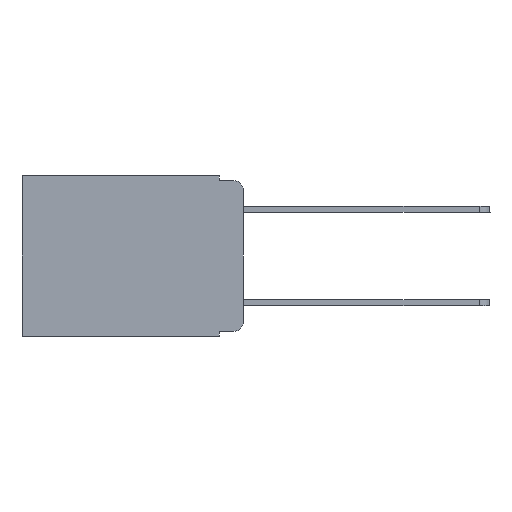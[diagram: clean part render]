
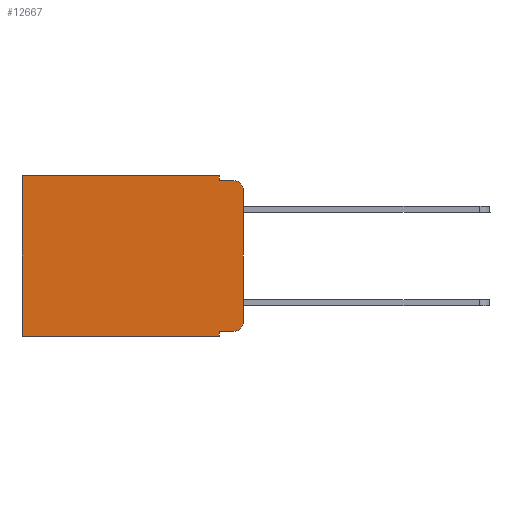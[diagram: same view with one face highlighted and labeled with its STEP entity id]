
A CAD part, left-side view. The second image highlights one B-rep face of the part: STEP entity #12667.
In plain terms, the highlighted planar face has unit normal (-1, 0, 0).
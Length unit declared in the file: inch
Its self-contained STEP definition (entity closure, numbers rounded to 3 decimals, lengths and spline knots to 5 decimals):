
#111 = CIRCLE ( 'NONE', #2934, 0.02 ) ;
#188 = ORIENTED_EDGE ( 'NONE', *, *, #13319, .T. ) ;
#190 = CIRCLE ( 'NONE', #20219, 0.02 ) ;
#275 = LINE ( 'NONE', #2709, #3419 ) ;
#318 = VERTEX_POINT ( 'NONE', #12634 ) ;
#684 = CARTESIAN_POINT ( 'NONE',  ( 0.298, 0.051, -0.333 ) ) ;
#744 = EDGE_CURVE ( 'NONE', #5972, #11045, #20165, .T. ) ;
#1204 = VECTOR ( 'NONE', #13060, 39.37008 ) ;
#1580 = CARTESIAN_POINT ( 'NONE',  ( 0.298, 0.051, 0. ) ) ;
#1635 = CARTESIAN_POINT ( 'NONE',  ( 0.298, 0., -0.343 ) ) ;
#1804 = DIRECTION ( 'NONE',  ( 0., 0., -1. ) ) ;
#1850 = LINE ( 'NONE', #1635, #4973 ) ;
#1986 = VERTEX_POINT ( 'NONE', #684 ) ;
#2709 = CARTESIAN_POINT ( 'NONE',  ( 0.298, 0.051, -0.333 ) ) ;
#2934 = AXIS2_PLACEMENT_3D ( 'NONE', #17163, #17082, #4686 ) ;
#3065 = CARTESIAN_POINT ( 'NONE',  ( 0.298, 0.02, -0.01 ) ) ;
#3326 = CARTESIAN_POINT ( 'NONE',  ( 0.298, 0., 0. ) ) ;
#3419 = VECTOR ( 'NONE', #6190, 39.37008 ) ;
#4187 = EDGE_CURVE ( 'NONE', #19024, #15727, #15552, .T. ) ;
#4202 = VECTOR ( 'NONE', #8834, 39.37008 ) ;
#4479 = FACE_OUTER_BOUND ( 'NONE', #5883, .T. ) ;
#4686 = DIRECTION ( 'NONE',  ( 0., 0., -1. ) ) ;
#4766 = AXIS2_PLACEMENT_3D ( 'NONE', #19698, #8995, #1804 ) ;
#4973 = VECTOR ( 'NONE', #15931, 39.37008 ) ;
#5771 = EDGE_CURVE ( 'NONE', #1986, #19850, #275, .T. ) ;
#5883 = EDGE_LOOP ( 'NONE', ( #16568, #188, #13346, #12240, #8488, #14328, #14435, #6673, #20327, #23247 ) ) ;
#5972 = VERTEX_POINT ( 'NONE', #1580 ) ;
#6190 = DIRECTION ( 'NONE',  ( 0., -1., 0. ) ) ;
#6331 = EDGE_CURVE ( 'NONE', #5972, #19024, #22505, .T. ) ;
#6673 = ORIENTED_EDGE ( 'NONE', *, *, #8323, .F. ) ;
#6708 = EDGE_CURVE ( 'NONE', #20943, #9662, #15771, .T. ) ;
#6944 = DIRECTION ( 'NONE',  ( 0., 0., -1. ) ) ;
#7244 = DIRECTION ( 'NONE',  ( 0., 0., -1. ) ) ;
#7416 = CARTESIAN_POINT ( 'NONE',  ( 0.298, 0., -0.313 ) ) ;
#7608 = CARTESIAN_POINT ( 'NONE',  ( 0.298, 0.473, 0. ) ) ;
#8323 = EDGE_CURVE ( 'NONE', #1986, #12819, #11779, .T. ) ;
#8488 = ORIENTED_EDGE ( 'NONE', *, *, #744, .T. ) ;
#8834 = DIRECTION ( 'NONE',  ( 0., 1., 0. ) ) ;
#8995 = DIRECTION ( 'NONE',  ( 1., 0., 0. ) ) ;
#9658 = CARTESIAN_POINT ( 'NONE',  ( 0.298, 0.051, -0.343 ) ) ;
#9662 = VERTEX_POINT ( 'NONE', #7416 ) ;
#10118 = DIRECTION ( 'NONE',  ( 0., 0., -1. ) ) ;
#10312 = EDGE_CURVE ( 'NONE', #12819, #318, #1850, .T. ) ;
#11045 = VERTEX_POINT ( 'NONE', #13282 ) ;
#11590 = VECTOR ( 'NONE', #7244, 39.37008 ) ;
#11779 = LINE ( 'NONE', #19026, #13176 ) ;
#12222 = CARTESIAN_POINT ( 'NONE',  ( 0.298, 0.051, -0.01 ) ) ;
#12240 = ORIENTED_EDGE ( 'NONE', *, *, #6331, .F. ) ;
#12578 = DIRECTION ( 'NONE',  ( -1., 0., 0. ) ) ;
#12582 = PLANE ( 'NONE',  #4766 ) ;
#12634 = CARTESIAN_POINT ( 'NONE',  ( 0.298, 0.473, -0.343 ) ) ;
#12667 = ADVANCED_FACE ( 'NONE', ( #4479 ), #12582, .F. ) ;
#12782 = DIRECTION ( 'NONE',  ( 0., 0., -1. ) ) ;
#12819 = VERTEX_POINT ( 'NONE', #9658 ) ;
#13060 = DIRECTION ( 'NONE',  ( 0., -1., 0. ) ) ;
#13176 = VECTOR ( 'NONE', #10118, 39.37008 ) ;
#13263 = VECTOR ( 'NONE', #15319, 39.37008 ) ;
#13282 = CARTESIAN_POINT ( 'NONE',  ( 0.298, 0.473, 0. ) ) ;
#13319 = EDGE_CURVE ( 'NONE', #20943, #15727, #190, .T. ) ;
#13346 = ORIENTED_EDGE ( 'NONE', *, *, #4187, .F. ) ;
#13872 = VECTOR ( 'NONE', #12782, 39.37008 ) ;
#14328 = ORIENTED_EDGE ( 'NONE', *, *, #16664, .T. ) ;
#14435 = ORIENTED_EDGE ( 'NONE', *, *, #10312, .F. ) ;
#15319 = DIRECTION ( 'NONE',  ( 0., 0., -1. ) ) ;
#15552 = LINE ( 'NONE', #18535, #1204 ) ;
#15727 = VERTEX_POINT ( 'NONE', #3065 ) ;
#15771 = LINE ( 'NONE', #17883, #11590 ) ;
#15931 = DIRECTION ( 'NONE',  ( 0., 1., 0. ) ) ;
#15963 = CARTESIAN_POINT ( 'NONE',  ( 0.298, 0.02, -0.333 ) ) ;
#16568 = ORIENTED_EDGE ( 'NONE', *, *, #6708, .F. ) ;
#16664 = EDGE_CURVE ( 'NONE', #11045, #318, #20864, .T. ) ;
#17082 = DIRECTION ( 'NONE',  ( -1., 0., 0. ) ) ;
#17163 = CARTESIAN_POINT ( 'NONE',  ( 0.298, 0.02, -0.313 ) ) ;
#17476 = CARTESIAN_POINT ( 'NONE',  ( 0.298, 0., -0.03 ) ) ;
#17883 = CARTESIAN_POINT ( 'NONE',  ( 0.298, 0., 0. ) ) ;
#18535 = CARTESIAN_POINT ( 'NONE',  ( 0.298, 0.051, -0.01 ) ) ;
#19024 = VERTEX_POINT ( 'NONE', #12222 ) ;
#19026 = CARTESIAN_POINT ( 'NONE',  ( 0.298, 0.051, 0. ) ) ;
#19698 = CARTESIAN_POINT ( 'NONE',  ( 0.298, 0., 0. ) ) ;
#19850 = VERTEX_POINT ( 'NONE', #15963 ) ;
#20165 = LINE ( 'NONE', #3326, #4202 ) ;
#20219 = AXIS2_PLACEMENT_3D ( 'NONE', #23129, #12578, #6944 ) ;
#20327 = ORIENTED_EDGE ( 'NONE', *, *, #5771, .T. ) ;
#20864 = LINE ( 'NONE', #7608, #13872 ) ;
#20943 = VERTEX_POINT ( 'NONE', #17476 ) ;
#21489 = EDGE_CURVE ( 'NONE', #19850, #9662, #111, .T. ) ;
#22442 = CARTESIAN_POINT ( 'NONE',  ( 0.298, 0.051, 0. ) ) ;
#22505 = LINE ( 'NONE', #22442, #13263 ) ;
#23129 = CARTESIAN_POINT ( 'NONE',  ( 0.298, 0.02, -0.03 ) ) ;
#23247 = ORIENTED_EDGE ( 'NONE', *, *, #21489, .T. ) ;
